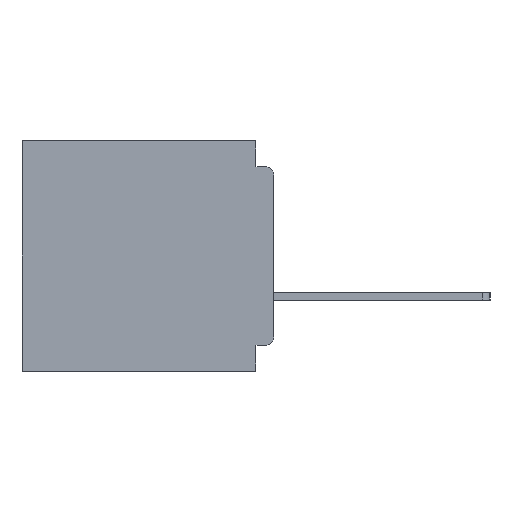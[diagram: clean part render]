
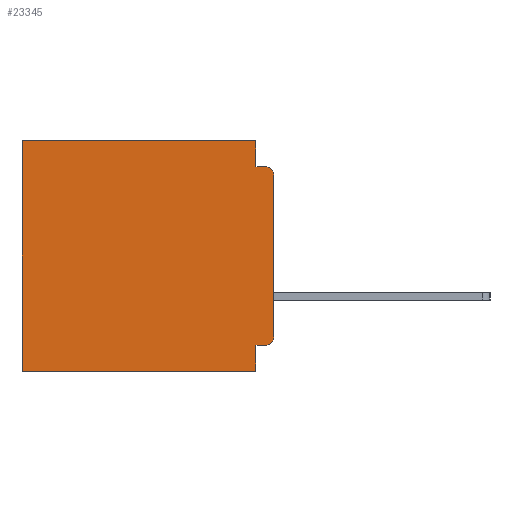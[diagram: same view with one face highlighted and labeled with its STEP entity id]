
A CAD part, left-side view. The second image highlights one B-rep face of the part: STEP entity #23345.
In plain terms, the highlighted planar face has unit normal (-1, 0, 0).
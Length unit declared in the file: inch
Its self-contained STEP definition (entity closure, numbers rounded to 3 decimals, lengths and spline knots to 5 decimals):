
#1421 = DIRECTION ( 'NONE',  ( 1., 0., 0. ) ) ;
#1796 = CARTESIAN_POINT ( 'NONE',  ( 0.3, 0.031, 0. ) ) ;
#1842 = CARTESIAN_POINT ( 'NONE',  ( 0.3, 0.015, -0.06 ) ) ;
#2042 = VERTEX_POINT ( 'NONE', #40366 ) ;
#3044 = CARTESIAN_POINT ( 'NONE',  ( 0.3, 0., -0.355 ) ) ;
#3444 = EDGE_LOOP ( 'NONE', ( #55083, #53625, #31909, #3546, #29057, #19670, #19691, #24194, #49642, #53250 ) ) ;
#3546 = ORIENTED_EDGE ( 'NONE', *, *, #42756, .F. ) ;
#4209 = AXIS2_PLACEMENT_3D ( 'NONE', #37780, #11914, #42093 ) ;
#4993 = EDGE_CURVE ( 'NONE', #5905, #39871, #26724, .T. ) ;
#5355 = PLANE ( 'NONE',  #39463 ) ;
#5905 = VERTEX_POINT ( 'NONE', #1796 ) ;
#6152 = DIRECTION ( 'NONE',  ( 0., 0., -1. ) ) ;
#7227 = CARTESIAN_POINT ( 'NONE',  ( 0.3, 0., -0.4 ) ) ;
#8646 = CARTESIAN_POINT ( 'NONE',  ( 0.3, 0.437, -0.4 ) ) ;
#9584 = EDGE_CURVE ( 'NONE', #2042, #42816, #14785, .T. ) ;
#9595 = LINE ( 'NONE', #35604, #12277 ) ;
#9752 = DIRECTION ( 'NONE',  ( 0., -1., 0. ) ) ;
#9859 = CARTESIAN_POINT ( 'NONE',  ( 0.3, 0., -0.4 ) ) ;
#10509 = VERTEX_POINT ( 'NONE', #44379 ) ;
#11914 = DIRECTION ( 'NONE',  ( -1., 0., 0. ) ) ;
#12277 = VECTOR ( 'NONE', #9752, 39.37008 ) ;
#13575 = VECTOR ( 'NONE', #37811, 39.37008 ) ;
#14200 = VECTOR ( 'NONE', #28556, 39.37008 ) ;
#14785 = LINE ( 'NONE', #7227, #14200 ) ;
#15221 = VERTEX_POINT ( 'NONE', #31816 ) ;
#16097 = DIRECTION ( 'NONE',  ( 0., 1., 0. ) ) ;
#16289 = LINE ( 'NONE', #33488, #13575 ) ;
#16449 = VERTEX_POINT ( 'NONE', #32058 ) ;
#16579 = VECTOR ( 'NONE', #37764, 39.37008 ) ;
#17316 = EDGE_CURVE ( 'NONE', #18531, #42816, #53490, .T. ) ;
#17692 = CARTESIAN_POINT ( 'NONE',  ( 0.3, 0.015, -0.045 ) ) ;
#18305 = EDGE_CURVE ( 'NONE', #39871, #10509, #36897, .T. ) ;
#18531 = VERTEX_POINT ( 'NONE', #44510 ) ;
#19032 = CARTESIAN_POINT ( 'NONE',  ( 0.3, 0.437, 0. ) ) ;
#19670 = ORIENTED_EDGE ( 'NONE', *, *, #18305, .T. ) ;
#19691 = ORIENTED_EDGE ( 'NONE', *, *, #23001, .F. ) ;
#20771 = CARTESIAN_POINT ( 'NONE',  ( 0.3, 0., -0.34 ) ) ;
#22939 = VECTOR ( 'NONE', #33215, 39.37008 ) ;
#23001 = EDGE_CURVE ( 'NONE', #25023, #10509, #49507, .T. ) ;
#23345 = ADVANCED_FACE ( 'NONE', ( #44846 ), #5355, .F. ) ;
#24010 = VECTOR ( 'NONE', #47289, 39.37008 ) ;
#24194 = ORIENTED_EDGE ( 'NONE', *, *, #40384, .F. ) ;
#25023 = VERTEX_POINT ( 'NONE', #27781 ) ;
#25230 = VECTOR ( 'NONE', #39956, 39.37008 ) ;
#26281 = EDGE_CURVE ( 'NONE', #2042, #54098, #28438, .T. ) ;
#26724 = LINE ( 'NONE', #37831, #16579 ) ;
#27781 = CARTESIAN_POINT ( 'NONE',  ( 0.3, 0.031, -0.4 ) ) ;
#28438 = CIRCLE ( 'NONE', #54313, 0.015 ) ;
#28556 = DIRECTION ( 'NONE',  ( 0., 0., -1. ) ) ;
#29057 = ORIENTED_EDGE ( 'NONE', *, *, #4993, .T. ) ;
#29173 = CARTESIAN_POINT ( 'NONE',  ( 0.3, 0., -0.4 ) ) ;
#31569 = DIRECTION ( 'NONE',  ( 0., 0., -1. ) ) ;
#31632 = EDGE_CURVE ( 'NONE', #16449, #54098, #9595, .T. ) ;
#31816 = CARTESIAN_POINT ( 'NONE',  ( 0.3, 0.031, -0.355 ) ) ;
#31909 = ORIENTED_EDGE ( 'NONE', *, *, #31632, .F. ) ;
#32001 = DIRECTION ( 'NONE',  ( -1., 0., 0. ) ) ;
#32058 = CARTESIAN_POINT ( 'NONE',  ( 0.3, 0.031, -0.045 ) ) ;
#33138 = LINE ( 'NONE', #3044, #22939 ) ;
#33215 = DIRECTION ( 'NONE',  ( 0., 1., 0. ) ) ;
#33488 = CARTESIAN_POINT ( 'NONE',  ( 0.3, 0.031, 0. ) ) ;
#35604 = CARTESIAN_POINT ( 'NONE',  ( 0.3, 0., -0.045 ) ) ;
#35633 = CARTESIAN_POINT ( 'NONE',  ( 0.3, 0.031, -0.4 ) ) ;
#36897 = LINE ( 'NONE', #8646, #24010 ) ;
#36916 = VECTOR ( 'NONE', #16097, 39.37008 ) ;
#37764 = DIRECTION ( 'NONE',  ( 0., 1., 0. ) ) ;
#37780 = CARTESIAN_POINT ( 'NONE',  ( 0.3, 0.015, -0.34 ) ) ;
#37811 = DIRECTION ( 'NONE',  ( 0., 0., -1. ) ) ;
#37831 = CARTESIAN_POINT ( 'NONE',  ( 0.3, 0., 0. ) ) ;
#38251 = EDGE_CURVE ( 'NONE', #18531, #15221, #33138, .T. ) ;
#39463 = AXIS2_PLACEMENT_3D ( 'NONE', #9859, #1421, #31569 ) ;
#39871 = VERTEX_POINT ( 'NONE', #19032 ) ;
#39956 = DIRECTION ( 'NONE',  ( 0., 0., -1. ) ) ;
#40366 = CARTESIAN_POINT ( 'NONE',  ( 0.3, 0., -0.06 ) ) ;
#40384 = EDGE_CURVE ( 'NONE', #15221, #25023, #49350, .T. ) ;
#42093 = DIRECTION ( 'NONE',  ( 0., 0., -1. ) ) ;
#42756 = EDGE_CURVE ( 'NONE', #5905, #16449, #16289, .T. ) ;
#42816 = VERTEX_POINT ( 'NONE', #20771 ) ;
#44379 = CARTESIAN_POINT ( 'NONE',  ( 0.3, 0.437, -0.4 ) ) ;
#44510 = CARTESIAN_POINT ( 'NONE',  ( 0.3, 0.015, -0.355 ) ) ;
#44846 = FACE_OUTER_BOUND ( 'NONE', #3444, .T. ) ;
#47289 = DIRECTION ( 'NONE',  ( 0., 0., -1. ) ) ;
#49350 = LINE ( 'NONE', #35633, #25230 ) ;
#49507 = LINE ( 'NONE', #29173, #36916 ) ;
#49642 = ORIENTED_EDGE ( 'NONE', *, *, #38251, .F. ) ;
#53250 = ORIENTED_EDGE ( 'NONE', *, *, #17316, .T. ) ;
#53490 = CIRCLE ( 'NONE', #4209, 0.015 ) ;
#53625 = ORIENTED_EDGE ( 'NONE', *, *, #26281, .T. ) ;
#54098 = VERTEX_POINT ( 'NONE', #17692 ) ;
#54313 = AXIS2_PLACEMENT_3D ( 'NONE', #1842, #32001, #6152 ) ;
#55083 = ORIENTED_EDGE ( 'NONE', *, *, #9584, .F. ) ;
